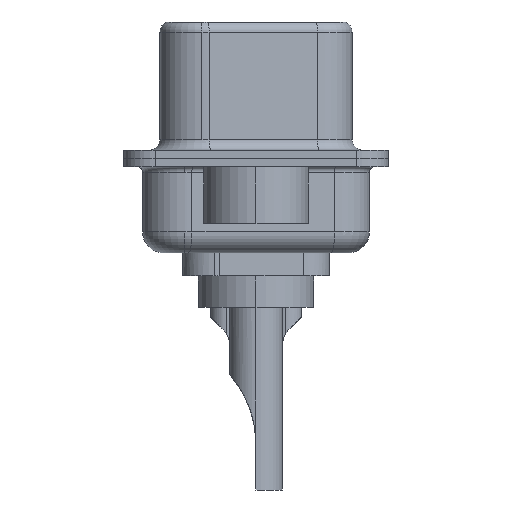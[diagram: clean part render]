
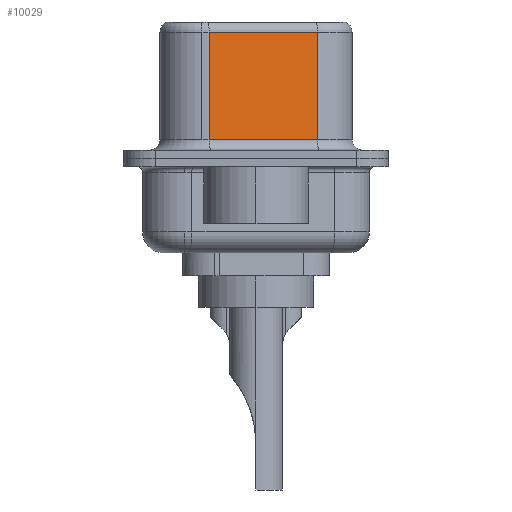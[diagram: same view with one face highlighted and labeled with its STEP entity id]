
A CAD part, left-side view. The second image highlights one B-rep face of the part: STEP entity #10029.
In plain terms, the highlighted planar face has unit normal (-0.985, -0.174, 0).
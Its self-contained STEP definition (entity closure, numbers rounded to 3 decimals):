
#58 = DIRECTION ( 'NONE',  ( 0., 0., -1. ) ) ;
#887 = EDGE_CURVE ( 'NONE', #7093, #12031, #4607, .T. ) ;
#1071 = VECTOR ( 'NONE', #17029, 1000. ) ;
#1685 = CARTESIAN_POINT ( 'NONE',  ( 4.565, -2.927, 0.9 ) ) ;
#2219 = DIRECTION ( 'NONE',  ( -0.174, 0.985, 0. ) ) ;
#3574 = EDGE_CURVE ( 'NONE', #5812, #5110, #8454, .T. ) ;
#3644 = AXIS2_PLACEMENT_3D ( 'NONE', #8212, #11124, #2219 ) ;
#3683 = PLANE ( 'NONE',  #3644 ) ;
#4607 = LINE ( 'NONE', #11294, #8552 ) ;
#5110 = VERTEX_POINT ( 'NONE', #18474 ) ;
#5812 = VERTEX_POINT ( 'NONE', #10709 ) ;
#7093 = VERTEX_POINT ( 'NONE', #12418 ) ;
#8138 = DIRECTION ( 'NONE',  ( -0.174, 0.985, 0. ) ) ;
#8176 = ORIENTED_EDGE ( 'NONE', *, *, #18674, .F. ) ;
#8212 = CARTESIAN_POINT ( 'NONE',  ( 4.565, -2.927, 6.52 ) ) ;
#8454 = LINE ( 'NONE', #11533, #11390 ) ;
#8552 = VECTOR ( 'NONE', #10778, 1000. ) ;
#9068 = LINE ( 'NONE', #15674, #1071 ) ;
#10029 = ADVANCED_FACE ( 'NONE', ( #12366 ), #3683, .F. ) ;
#10709 = CARTESIAN_POINT ( 'NONE',  ( 4.565, -2.927, 6.02 ) ) ;
#10778 = DIRECTION ( 'NONE',  ( 0.174, -0.985, 0. ) ) ;
#11124 = DIRECTION ( 'NONE',  ( 0.985, 0.174, 0. ) ) ;
#11294 = CARTESIAN_POINT ( 'NONE',  ( 4.565, -2.927, 0.9 ) ) ;
#11390 = VECTOR ( 'NONE', #8138, 1000. ) ;
#11533 = CARTESIAN_POINT ( 'NONE',  ( 4.565, -2.927, 6.02 ) ) ;
#12031 = VERTEX_POINT ( 'NONE', #1685 ) ;
#12366 = FACE_OUTER_BOUND ( 'NONE', #12561, .T. ) ;
#12418 = CARTESIAN_POINT ( 'NONE',  ( 3.655, 2.233, 0.9 ) ) ;
#12561 = EDGE_LOOP ( 'NONE', ( #8176, #16000, #16638, #14111 ) ) ;
#13196 = VECTOR ( 'NONE', #58, 1000. ) ;
#13308 = EDGE_CURVE ( 'NONE', #5110, #7093, #9068, .T. ) ;
#13659 = LINE ( 'NONE', #16094, #13196 ) ;
#14111 = ORIENTED_EDGE ( 'NONE', *, *, #887, .T. ) ;
#15674 = CARTESIAN_POINT ( 'NONE',  ( 3.655, 2.233, 6.52 ) ) ;
#16000 = ORIENTED_EDGE ( 'NONE', *, *, #3574, .T. ) ;
#16094 = CARTESIAN_POINT ( 'NONE',  ( 4.565, -2.927, 6.52 ) ) ;
#16638 = ORIENTED_EDGE ( 'NONE', *, *, #13308, .T. ) ;
#17029 = DIRECTION ( 'NONE',  ( 0., 0., -1. ) ) ;
#18474 = CARTESIAN_POINT ( 'NONE',  ( 3.655, 2.233, 6.02 ) ) ;
#18674 = EDGE_CURVE ( 'NONE', #5812, #12031, #13659, .T. ) ;
